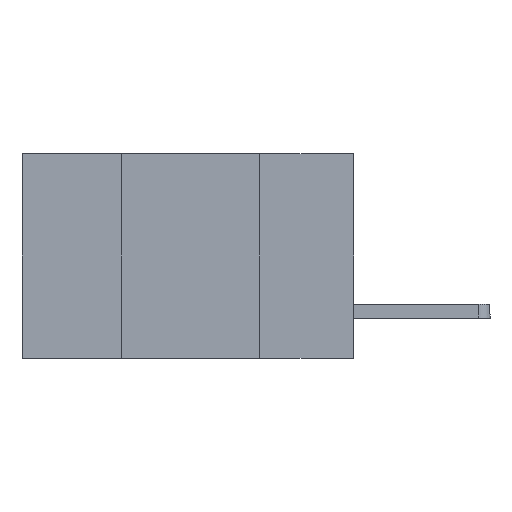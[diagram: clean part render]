
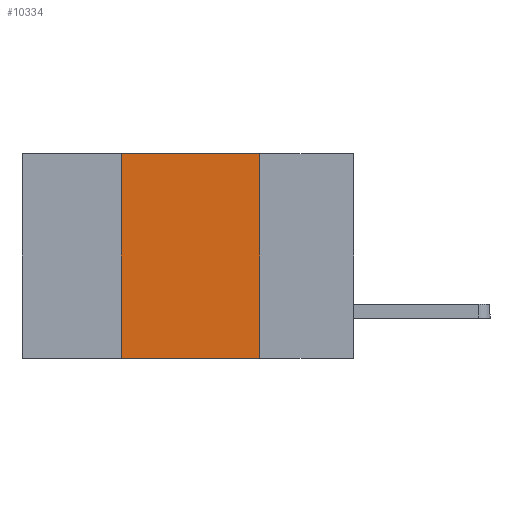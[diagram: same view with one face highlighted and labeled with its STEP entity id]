
A CAD part, left-side view. The second image highlights one B-rep face of the part: STEP entity #10334.
In plain terms, the highlighted planar face has unit normal (-1, 0, 0).
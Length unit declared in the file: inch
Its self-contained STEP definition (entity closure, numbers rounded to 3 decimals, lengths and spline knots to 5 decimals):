
#846 = PLANE ( 'NONE',  #10160 ) ;
#1101 = VECTOR ( 'NONE', #11538, 39.37008 ) ;
#1274 = EDGE_LOOP ( 'NONE', ( #10610, #10044, #6643, #2521 ) ) ;
#1529 = FACE_OUTER_BOUND ( 'NONE', #1274, .T. ) ;
#2287 = VECTOR ( 'NONE', #7354, 39.37008 ) ;
#2501 = VERTEX_POINT ( 'NONE', #11093 ) ;
#2521 = ORIENTED_EDGE ( 'NONE', *, *, #11638, .T. ) ;
#2614 = CARTESIAN_POINT ( 'NONE',  ( 0., 0.6, 0. ) ) ;
#2907 = LINE ( 'NONE', #11683, #2287 ) ;
#3406 = LINE ( 'NONE', #2614, #1101 ) ;
#3964 = EDGE_CURVE ( 'NONE', #2501, #5157, #6999, .T. ) ;
#4706 = DIRECTION ( 'NONE',  ( 1., 0., 0. ) ) ;
#5150 = EDGE_CURVE ( 'NONE', #8365, #8358, #6824, .T. ) ;
#5157 = VERTEX_POINT ( 'NONE', #11534 ) ;
#5343 = CARTESIAN_POINT ( 'NONE',  ( 0., 0.42, 0. ) ) ;
#6175 = CARTESIAN_POINT ( 'NONE',  ( 0., 0.42, -0.37 ) ) ;
#6324 = DIRECTION ( 'NONE',  ( 0., 0., 1. ) ) ;
#6643 = ORIENTED_EDGE ( 'NONE', *, *, #5150, .F. ) ;
#6824 = LINE ( 'NONE', #5343, #8920 ) ;
#6999 = LINE ( 'NONE', #7445, #11336 ) ;
#7354 = DIRECTION ( 'NONE',  ( 0., -1., 0. ) ) ;
#7445 = CARTESIAN_POINT ( 'NONE',  ( 0., 0.17, 0. ) ) ;
#7930 = CARTESIAN_POINT ( 'NONE',  ( 0., 0.42, 0. ) ) ;
#8349 = DIRECTION ( 'NONE',  ( 0., 0., -1. ) ) ;
#8358 = VERTEX_POINT ( 'NONE', #7930 ) ;
#8365 = VERTEX_POINT ( 'NONE', #6175 ) ;
#8920 = VECTOR ( 'NONE', #6324, 39.37008 ) ;
#10044 = ORIENTED_EDGE ( 'NONE', *, *, #10207, .F. ) ;
#10109 = CARTESIAN_POINT ( 'NONE',  ( 0., 0.6, 0. ) ) ;
#10160 = AXIS2_PLACEMENT_3D ( 'NONE', #10109, #4706, #10930 ) ;
#10207 = EDGE_CURVE ( 'NONE', #8358, #2501, #3406, .T. ) ;
#10334 = ADVANCED_FACE ( 'NONE', ( #1529 ), #846, .F. ) ;
#10610 = ORIENTED_EDGE ( 'NONE', *, *, #3964, .F. ) ;
#10930 = DIRECTION ( 'NONE',  ( 0., 0., -1. ) ) ;
#11093 = CARTESIAN_POINT ( 'NONE',  ( 0., 0.17, 0. ) ) ;
#11336 = VECTOR ( 'NONE', #8349, 39.37008 ) ;
#11534 = CARTESIAN_POINT ( 'NONE',  ( 0., 0.17, -0.37 ) ) ;
#11538 = DIRECTION ( 'NONE',  ( 0., -1., 0. ) ) ;
#11638 = EDGE_CURVE ( 'NONE', #8365, #5157, #2907, .T. ) ;
#11683 = CARTESIAN_POINT ( 'NONE',  ( 0., 0.6, -0.37 ) ) ;
